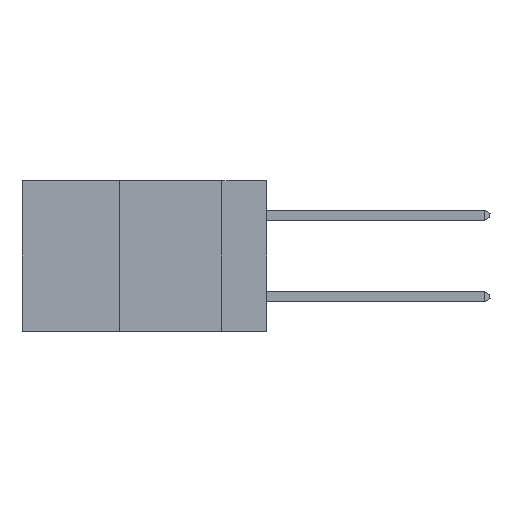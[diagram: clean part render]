
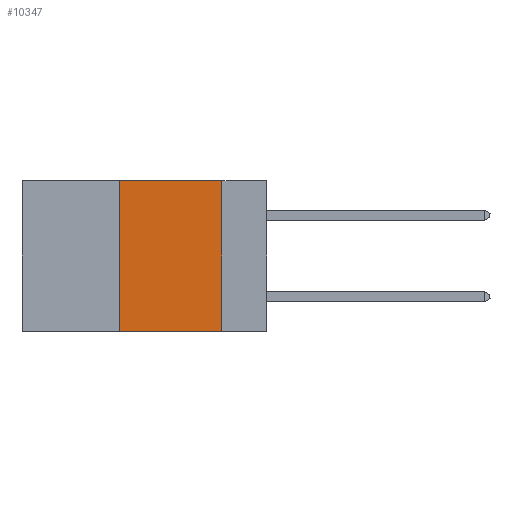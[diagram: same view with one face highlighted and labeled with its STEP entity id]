
A CAD part, left-side view. The second image highlights one B-rep face of the part: STEP entity #10347.
In plain terms, the highlighted planar face has unit normal (-1, 0, 0).
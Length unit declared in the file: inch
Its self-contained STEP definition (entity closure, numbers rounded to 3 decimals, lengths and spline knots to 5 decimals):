
#124 = LINE ( 'NONE', #4817, #11399 ) ;
#500 = EDGE_LOOP ( 'NONE', ( #6048, #5146, #2736, #5975 ) ) ;
#634 = VERTEX_POINT ( 'NONE', #13254 ) ;
#972 = EDGE_CURVE ( 'NONE', #634, #9074, #9803, .T. ) ;
#1365 = DIRECTION ( 'NONE',  ( 0., 0., -1. ) ) ;
#1687 = PLANE ( 'NONE',  #12622 ) ;
#1910 = CARTESIAN_POINT ( 'NONE',  ( 0., 0.11, -0.37 ) ) ;
#2468 = VECTOR ( 'NONE', #7137, 39.37008 ) ;
#2736 = ORIENTED_EDGE ( 'NONE', *, *, #972, .F. ) ;
#2995 = DIRECTION ( 'NONE',  ( 1., 0., 0. ) ) ;
#3887 = CARTESIAN_POINT ( 'NONE',  ( 0., 0.6, -0.37 ) ) ;
#4408 = EDGE_CURVE ( 'NONE', #9074, #5599, #11654, .T. ) ;
#4817 = CARTESIAN_POINT ( 'NONE',  ( 0., 0.11, 0. ) ) ;
#5146 = ORIENTED_EDGE ( 'NONE', *, *, #4408, .F. ) ;
#5517 = EDGE_CURVE ( 'NONE', #634, #9087, #6251, .T. ) ;
#5599 = VERTEX_POINT ( 'NONE', #13763 ) ;
#5975 = ORIENTED_EDGE ( 'NONE', *, *, #5517, .T. ) ;
#5989 = CARTESIAN_POINT ( 'NONE',  ( 0., 0.6, 0. ) ) ;
#6048 = ORIENTED_EDGE ( 'NONE', *, *, #9472, .F. ) ;
#6251 = LINE ( 'NONE', #3887, #8640 ) ;
#6385 = VECTOR ( 'NONE', #8139, 39.37008 ) ;
#7137 = DIRECTION ( 'NONE',  ( 0., 0., 1. ) ) ;
#8139 = DIRECTION ( 'NONE',  ( 0., -1., 0. ) ) ;
#8640 = VECTOR ( 'NONE', #11693, 39.37008 ) ;
#9074 = VERTEX_POINT ( 'NONE', #13912 ) ;
#9087 = VERTEX_POINT ( 'NONE', #1910 ) ;
#9472 = EDGE_CURVE ( 'NONE', #5599, #9087, #124, .T. ) ;
#9803 = LINE ( 'NONE', #10279, #2468 ) ;
#10023 = FACE_OUTER_BOUND ( 'NONE', #500, .T. ) ;
#10279 = CARTESIAN_POINT ( 'NONE',  ( 0., 0.36, 0. ) ) ;
#10347 = ADVANCED_FACE ( 'NONE', ( #10023 ), #1687, .F. ) ;
#11399 = VECTOR ( 'NONE', #1365, 39.37008 ) ;
#11591 = CARTESIAN_POINT ( 'NONE',  ( 0., 0.6, 0. ) ) ;
#11654 = LINE ( 'NONE', #5989, #6385 ) ;
#11693 = DIRECTION ( 'NONE',  ( 0., -1., 0. ) ) ;
#12622 = AXIS2_PLACEMENT_3D ( 'NONE', #11591, #2995, #13768 ) ;
#13254 = CARTESIAN_POINT ( 'NONE',  ( 0., 0.36, -0.37 ) ) ;
#13763 = CARTESIAN_POINT ( 'NONE',  ( 0., 0.11, 0. ) ) ;
#13768 = DIRECTION ( 'NONE',  ( 0., 0., -1. ) ) ;
#13912 = CARTESIAN_POINT ( 'NONE',  ( 0., 0.36, 0. ) ) ;
